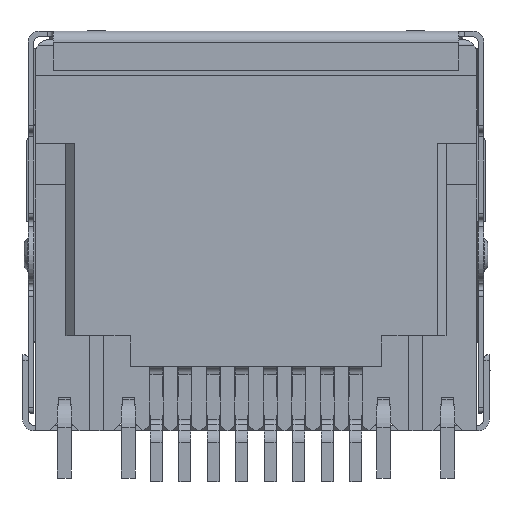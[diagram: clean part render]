
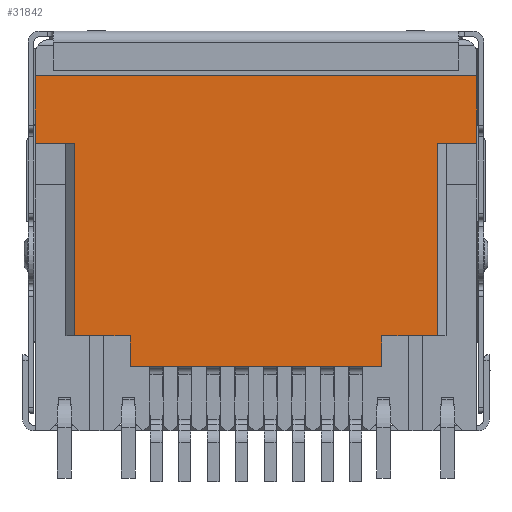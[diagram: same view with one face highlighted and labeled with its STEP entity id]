
A CAD part, front view. The second image highlights one B-rep face of the part: STEP entity #31842.
In plain terms, the highlighted planar face has unit normal (0, -1, 0).
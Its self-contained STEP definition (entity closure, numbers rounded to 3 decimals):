
#360 = VECTOR ( 'NONE', #26767, 1000. ) ;
#1020 = LINE ( 'NONE', #42525, #22814 ) ;
#1353 = DIRECTION ( 'NONE',  ( 0., 0., 1. ) ) ;
#1370 = EDGE_CURVE ( 'NONE', #40557, #48492, #1020, .T. ) ;
#1574 = DIRECTION ( 'NONE',  ( 1., 0., 0. ) ) ;
#1737 = CARTESIAN_POINT ( 'NONE',  ( -7.9, -5.525, -3.7 ) ) ;
#1858 = CARTESIAN_POINT ( 'NONE',  ( -7.9, -5.525, -14. ) ) ;
#2566 = EDGE_CURVE ( 'NONE', #27195, #21221, #34854, .T. ) ;
#3939 = LINE ( 'NONE', #8498, #12993 ) ;
#4006 = LINE ( 'NONE', #43607, #32525 ) ;
#4021 = VERTEX_POINT ( 'NONE', #7637 ) ;
#4087 = CARTESIAN_POINT ( 'NONE',  ( 4.5, -5.525, -10.6 ) ) ;
#4382 = LINE ( 'NONE', #43276, #31672 ) ;
#4556 = CARTESIAN_POINT ( 'NONE',  ( -7.9, -5.525, -1.3 ) ) ;
#5264 = VERTEX_POINT ( 'NONE', #7203 ) ;
#5333 = DIRECTION ( 'NONE',  ( 1., 0., 0. ) ) ;
#5492 = CARTESIAN_POINT ( 'NONE',  ( -7.9, -5.525, -3.7 ) ) ;
#5845 = ORIENTED_EDGE ( 'NONE', *, *, #1370, .T. ) ;
#6411 = DIRECTION ( 'NONE',  ( 1., 0., 0. ) ) ;
#6921 = ORIENTED_EDGE ( 'NONE', *, *, #46530, .T. ) ;
#7103 = EDGE_CURVE ( 'NONE', #5264, #40557, #42228, .T. ) ;
#7203 = CARTESIAN_POINT ( 'NONE',  ( 4.5, -5.525, -11.7 ) ) ;
#7268 = LINE ( 'NONE', #21241, #46125 ) ;
#7579 = ORIENTED_EDGE ( 'NONE', *, *, #7103, .T. ) ;
#7637 = CARTESIAN_POINT ( 'NONE',  ( 6.5, -5.525, -3.7 ) ) ;
#8278 = CARTESIAN_POINT ( 'NONE',  ( -7.9, -5.525, -11.7 ) ) ;
#8498 = CARTESIAN_POINT ( 'NONE',  ( -7.9, -5.525, -14. ) ) ;
#9153 = ORIENTED_EDGE ( 'NONE', *, *, #22995, .T. ) ;
#9521 = EDGE_CURVE ( 'NONE', #41220, #22944, #16089, .T. ) ;
#10225 = VERTEX_POINT ( 'NONE', #14522 ) ;
#11231 = DIRECTION ( 'NONE',  ( -1., 0., 0. ) ) ;
#12274 = CARTESIAN_POINT ( 'NONE',  ( -6.5, -5.525, -10.6 ) ) ;
#12350 = VECTOR ( 'NONE', #35420, 1000. ) ;
#12537 = DIRECTION ( 'NONE',  ( 0., 0., -1. ) ) ;
#12905 = LINE ( 'NONE', #5492, #40252 ) ;
#12993 = VECTOR ( 'NONE', #43302, 1000. ) ;
#14522 = CARTESIAN_POINT ( 'NONE',  ( -7.9, -5.525, -3.7 ) ) ;
#14638 = ORIENTED_EDGE ( 'NONE', *, *, #38929, .T. ) ;
#14680 = VERTEX_POINT ( 'NONE', #42605 ) ;
#16089 = LINE ( 'NONE', #28645, #17243 ) ;
#16320 = CARTESIAN_POINT ( 'NONE',  ( -4.5, -5.525, -11.7 ) ) ;
#17243 = VECTOR ( 'NONE', #36106, 1000. ) ;
#17676 = CARTESIAN_POINT ( 'NONE',  ( 6.5, -5.525, -10.6 ) ) ;
#17913 = ORIENTED_EDGE ( 'NONE', *, *, #23309, .F. ) ;
#18968 = EDGE_LOOP ( 'NONE', ( #14638, #17913, #39168, #46006, #27500, #22259, #39117, #9153, #26536, #7579, #5845, #6921 ) ) ;
#19352 = VERTEX_POINT ( 'NONE', #44365 ) ;
#19713 = EDGE_CURVE ( 'NONE', #10225, #21221, #3939, .T. ) ;
#20257 = VECTOR ( 'NONE', #11231, 1000. ) ;
#20321 = EDGE_CURVE ( 'NONE', #10225, #41220, #12905, .T. ) ;
#21221 = VERTEX_POINT ( 'NONE', #4556 ) ;
#21241 = CARTESIAN_POINT ( 'NONE',  ( -7.9, -5.525, -10.6 ) ) ;
#22259 = ORIENTED_EDGE ( 'NONE', *, *, #9521, .T. ) ;
#22814 = VECTOR ( 'NONE', #34382, 1000. ) ;
#22944 = VERTEX_POINT ( 'NONE', #12274 ) ;
#22995 = EDGE_CURVE ( 'NONE', #14680, #48759, #45618, .T. ) ;
#23309 = EDGE_CURVE ( 'NONE', #27195, #19352, #4382, .T. ) ;
#24559 = PLANE ( 'NONE',  #38635 ) ;
#25053 = DIRECTION ( 'NONE',  ( 0., -1., 0. ) ) ;
#25529 = VECTOR ( 'NONE', #43672, 1000. ) ;
#26536 = ORIENTED_EDGE ( 'NONE', *, *, #37042, .T. ) ;
#26767 = DIRECTION ( 'NONE',  ( 0., 0., 1. ) ) ;
#27195 = VERTEX_POINT ( 'NONE', #29405 ) ;
#27500 = ORIENTED_EDGE ( 'NONE', *, *, #20321, .T. ) ;
#28483 = CARTESIAN_POINT ( 'NONE',  ( -6.5, -5.525, -3.7 ) ) ;
#28645 = CARTESIAN_POINT ( 'NONE',  ( -6.5, -5.525, -14. ) ) ;
#28972 = DIRECTION ( 'NONE',  ( 0., 0., -1. ) ) ;
#29405 = CARTESIAN_POINT ( 'NONE',  ( 7.9, -5.525, -1.3 ) ) ;
#30813 = FACE_OUTER_BOUND ( 'NONE', #18968, .T. ) ;
#31672 = VECTOR ( 'NONE', #12537, 1000. ) ;
#31842 = ADVANCED_FACE ( 'NONE', ( #30813 ), #24559, .T. ) ;
#32525 = VECTOR ( 'NONE', #1353, 1000. ) ;
#32796 = CARTESIAN_POINT ( 'NONE',  ( 4.5, -5.525, -10.6 ) ) ;
#34382 = DIRECTION ( 'NONE',  ( 1., 0., 0. ) ) ;
#34854 = LINE ( 'NONE', #49924, #20257 ) ;
#35420 = DIRECTION ( 'NONE',  ( 1., 0., 0. ) ) ;
#36106 = DIRECTION ( 'NONE',  ( 0., 0., -1. ) ) ;
#37042 = EDGE_CURVE ( 'NONE', #48759, #5264, #39685, .T. ) ;
#38635 = AXIS2_PLACEMENT_3D ( 'NONE', #1858, #25053, #28972 ) ;
#38929 = EDGE_CURVE ( 'NONE', #4021, #19352, #43791, .T. ) ;
#39117 = ORIENTED_EDGE ( 'NONE', *, *, #43175, .T. ) ;
#39168 = ORIENTED_EDGE ( 'NONE', *, *, #2566, .T. ) ;
#39685 = LINE ( 'NONE', #8278, #12350 ) ;
#40252 = VECTOR ( 'NONE', #5333, 1000. ) ;
#40557 = VERTEX_POINT ( 'NONE', #32796 ) ;
#41220 = VERTEX_POINT ( 'NONE', #28483 ) ;
#42228 = LINE ( 'NONE', #4087, #360 ) ;
#42525 = CARTESIAN_POINT ( 'NONE',  ( -7.9, -5.525, -10.6 ) ) ;
#42605 = CARTESIAN_POINT ( 'NONE',  ( -4.5, -5.525, -10.6 ) ) ;
#43175 = EDGE_CURVE ( 'NONE', #22944, #14680, #7268, .T. ) ;
#43276 = CARTESIAN_POINT ( 'NONE',  ( 7.9, -5.525, -14. ) ) ;
#43302 = DIRECTION ( 'NONE',  ( 0., 0., 1. ) ) ;
#43607 = CARTESIAN_POINT ( 'NONE',  ( 6.5, -5.525, -14. ) ) ;
#43672 = DIRECTION ( 'NONE',  ( 0., 0., -1. ) ) ;
#43791 = LINE ( 'NONE', #1737, #49848 ) ;
#44365 = CARTESIAN_POINT ( 'NONE',  ( 7.9, -5.525, -3.7 ) ) ;
#45618 = LINE ( 'NONE', #47897, #25529 ) ;
#46006 = ORIENTED_EDGE ( 'NONE', *, *, #19713, .F. ) ;
#46125 = VECTOR ( 'NONE', #6411, 1000. ) ;
#46530 = EDGE_CURVE ( 'NONE', #48492, #4021, #4006, .T. ) ;
#47897 = CARTESIAN_POINT ( 'NONE',  ( -4.5, -5.525, -10.6 ) ) ;
#48492 = VERTEX_POINT ( 'NONE', #17676 ) ;
#48759 = VERTEX_POINT ( 'NONE', #16320 ) ;
#49848 = VECTOR ( 'NONE', #1574, 1000. ) ;
#49924 = CARTESIAN_POINT ( 'NONE',  ( -7.9, -5.525, -1.3 ) ) ;
